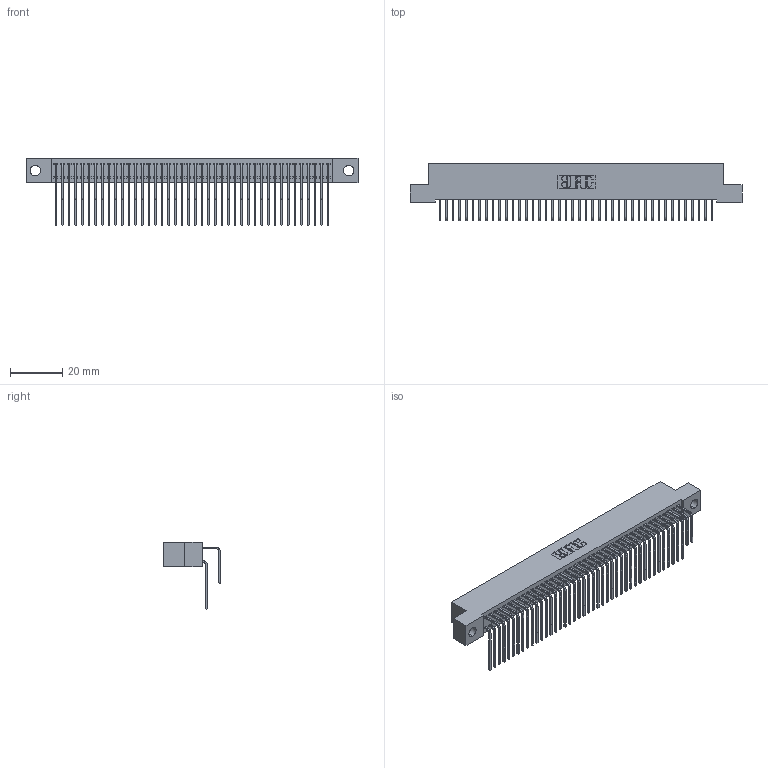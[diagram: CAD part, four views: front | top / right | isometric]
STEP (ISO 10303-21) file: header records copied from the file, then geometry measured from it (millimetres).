
FILE_DESCRIPTION (( 'STEP AP203' ), '1' );
FILE_NAME ('392-084-558-204.STEP', '2018-08-18T04:49:35', ( '' ), ( '' ), 'SwSTEP 2.0', 'SolidWorks 2016', '' );
FILE_SCHEMA (( 'CONFIG_CONTROL_DESIGN' ));
Length unit declared in the file: inch
Products named in the file (4): 342 Part_.156 TH; 345-292-001_558 559 Tail - 1; 345-292-001_558 Tail - 2; 392-084-558-204
Assembly tree (85 placements, depth 2):
  392-084-558-204
    342 Part_.156 TH
    345-292-001_558 559 Tail - 1  x42
    345-292-001_558 Tail - 2  x42
Bounding box: 127 x 21.91 x 25.78 mm (x, y, z)
Volume: 11808.5 mm3; surface area: 21237.5 mm2
Topology: 85 solids, 85 shells, 4646 faces, 13823 edges, 9102 vertices
Faces by surface type: plane 3258, cylinder 1388
Entity records: 28675 total; most frequent: CARTESIAN_POINT 4801, ORIENTED_EDGE 4686, DIRECTION 4083, EDGE_CURVE 2343, VECTOR 2175, LINE 2175, VERTEX_POINT 1558, AXIS2_PLACEMENT_3D 954
